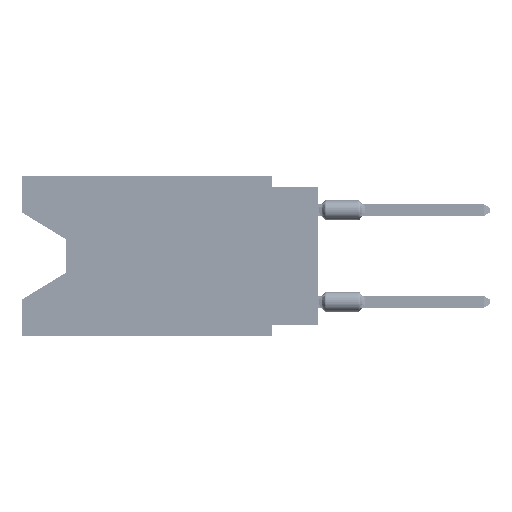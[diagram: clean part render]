
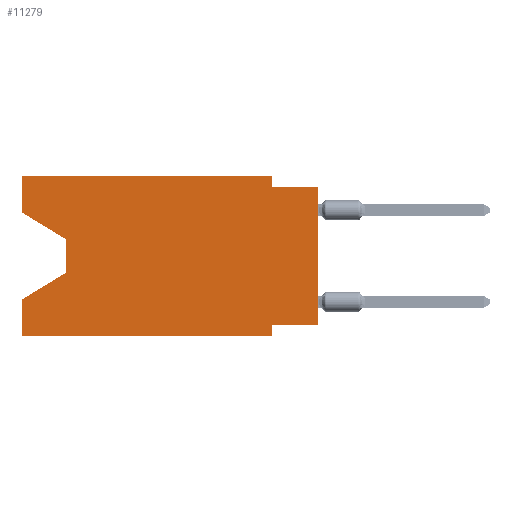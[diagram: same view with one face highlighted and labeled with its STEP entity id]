
A CAD part, left-side view. The second image highlights one B-rep face of the part: STEP entity #11279.
In plain terms, the highlighted planar face has unit normal (-1, 0, 0).
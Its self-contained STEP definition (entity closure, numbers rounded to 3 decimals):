
#950 = DIRECTION ( 'NONE',  ( 0., 0., 1. ) ) ;
#1279 = ORIENTED_EDGE ( 'NONE', *, *, #29455, .F. ) ;
#1303 = LINE ( 'NONE', #45888, #50963 ) ;
#3090 = CARTESIAN_POINT ( 'NONE',  ( 0., 16.383, -8.89 ) ) ;
#3572 = CARTESIAN_POINT ( 'NONE',  ( 0., 2.54, -8.89 ) ) ;
#4614 = VERTEX_POINT ( 'NONE', #33083 ) ;
#5511 = VECTOR ( 'NONE', #44005, 1000. ) ;
#6812 = CARTESIAN_POINT ( 'NONE',  ( 0., 0., -0.635 ) ) ;
#6932 = CARTESIAN_POINT ( 'NONE',  ( 0., 2.54, -8.89 ) ) ;
#8060 = EDGE_CURVE ( 'NONE', #33453, #52385, #30793, .T. ) ;
#8315 = LINE ( 'NONE', #13785, #61942 ) ;
#8865 = VECTOR ( 'NONE', #48893, 1000. ) ;
#9312 = VECTOR ( 'NONE', #46391, 1000. ) ;
#9789 = EDGE_CURVE ( 'NONE', #4614, #21553, #8315, .T. ) ;
#11019 = ORIENTED_EDGE ( 'NONE', *, *, #30261, .F. ) ;
#11279 = ADVANCED_FACE ( 'NONE', ( #70111 ), #65358, .F. ) ;
#13785 = CARTESIAN_POINT ( 'NONE',  ( 0., 16.383, -2.038 ) ) ;
#13865 = LINE ( 'NONE', #70539, #41864 ) ;
#14086 = EDGE_CURVE ( 'NONE', #66537, #68276, #41942, .T. ) ;
#14287 = DIRECTION ( 'NONE',  ( 0., 0., 1. ) ) ;
#15122 = CARTESIAN_POINT ( 'NONE',  ( 0., 16.383, 0. ) ) ;
#15493 = LINE ( 'NONE', #59031, #36379 ) ;
#15841 = LINE ( 'NONE', #71785, #44461 ) ;
#16662 = AXIS2_PLACEMENT_3D ( 'NONE', #71562, #37548, #26945 ) ;
#17237 = LINE ( 'NONE', #39890, #37788 ) ;
#18058 = LINE ( 'NONE', #53416, #25051 ) ;
#18403 = ORIENTED_EDGE ( 'NONE', *, *, #62581, .F. ) ;
#18841 = LINE ( 'NONE', #63453, #46507 ) ;
#19625 = VERTEX_POINT ( 'NONE', #66062 ) ;
#21553 = VERTEX_POINT ( 'NONE', #54909 ) ;
#21654 = ORIENTED_EDGE ( 'NONE', *, *, #52758, .F. ) ;
#21804 = CARTESIAN_POINT ( 'NONE',  ( 0., 13.97, -5.385 ) ) ;
#23381 = LINE ( 'NONE', #67645, #9312 ) ;
#24549 = VECTOR ( 'NONE', #53854, 1000. ) ;
#25051 = VECTOR ( 'NONE', #14287, 1000. ) ;
#25361 = DIRECTION ( 'NONE',  ( 0., 0., -1. ) ) ;
#26404 = VERTEX_POINT ( 'NONE', #3090 ) ;
#26851 = ORIENTED_EDGE ( 'NONE', *, *, #43022, .T. ) ;
#26939 = CARTESIAN_POINT ( 'NONE',  ( 0., 16.383, -6.852 ) ) ;
#26945 = DIRECTION ( 'NONE',  ( 0., 0., -1. ) ) ;
#28386 = ORIENTED_EDGE ( 'NONE', *, *, #14086, .F. ) ;
#28554 = VERTEX_POINT ( 'NONE', #26939 ) ;
#28732 = EDGE_CURVE ( 'NONE', #42422, #52385, #18841, .T. ) ;
#29455 = EDGE_CURVE ( 'NONE', #60139, #19625, #13865, .T. ) ;
#30261 = EDGE_CURVE ( 'NONE', #19625, #33453, #23381, .T. ) ;
#30793 = LINE ( 'NONE', #6812, #24549 ) ;
#33083 = CARTESIAN_POINT ( 'NONE',  ( 0., 16.383, -2.038 ) ) ;
#33453 = VERTEX_POINT ( 'NONE', #35591 ) ;
#34282 = VERTEX_POINT ( 'NONE', #21804 ) ;
#34705 = ORIENTED_EDGE ( 'NONE', *, *, #71980, .T. ) ;
#35591 = CARTESIAN_POINT ( 'NONE',  ( 0., 2.54, -0.635 ) ) ;
#36379 = VECTOR ( 'NONE', #25361, 1000. ) ;
#36411 = EDGE_CURVE ( 'NONE', #26404, #68276, #17237, .T. ) ;
#37548 = DIRECTION ( 'NONE',  ( 1., 0., 0. ) ) ;
#37788 = VECTOR ( 'NONE', #57103, 1000. ) ;
#38464 = CARTESIAN_POINT ( 'NONE',  ( 0., 2.54, -8.255 ) ) ;
#38511 = LINE ( 'NONE', #65253, #5511 ) ;
#39890 = CARTESIAN_POINT ( 'NONE',  ( 0., 16.383, -8.89 ) ) ;
#41864 = VECTOR ( 'NONE', #69451, 1000. ) ;
#41942 = LINE ( 'NONE', #3572, #8865 ) ;
#42422 = VERTEX_POINT ( 'NONE', #68024 ) ;
#43022 = EDGE_CURVE ( 'NONE', #34282, #28554, #38511, .T. ) ;
#44005 = DIRECTION ( 'NONE',  ( 0., 0.855, -0.519 ) ) ;
#44461 = VECTOR ( 'NONE', #55701, 1000. ) ;
#45888 = CARTESIAN_POINT ( 'NONE',  ( 0., 0., -8.255 ) ) ;
#46391 = DIRECTION ( 'NONE',  ( 0., 0., -1. ) ) ;
#46507 = VECTOR ( 'NONE', #950, 1000. ) ;
#46992 = ORIENTED_EDGE ( 'NONE', *, *, #36411, .T. ) ;
#47183 = EDGE_CURVE ( 'NONE', #4614, #60139, #15841, .T. ) ;
#47231 = ORIENTED_EDGE ( 'NONE', *, *, #8060, .F. ) ;
#48893 = DIRECTION ( 'NONE',  ( 0., 0., -1. ) ) ;
#50963 = VECTOR ( 'NONE', #68210, 1000. ) ;
#52385 = VERTEX_POINT ( 'NONE', #59495 ) ;
#52562 = DIRECTION ( 'NONE',  ( 0., -0.855, -0.519 ) ) ;
#52758 = EDGE_CURVE ( 'NONE', #42422, #66537, #1303, .T. ) ;
#53416 = CARTESIAN_POINT ( 'NONE',  ( 0., 16.383, 0. ) ) ;
#53854 = DIRECTION ( 'NONE',  ( 0., -1., 0. ) ) ;
#53979 = ORIENTED_EDGE ( 'NONE', *, *, #9789, .T. ) ;
#54909 = CARTESIAN_POINT ( 'NONE',  ( 0., 13.97, -3.505 ) ) ;
#55701 = DIRECTION ( 'NONE',  ( 0., 0., 1. ) ) ;
#57103 = DIRECTION ( 'NONE',  ( 0., -1., 0. ) ) ;
#57402 = ORIENTED_EDGE ( 'NONE', *, *, #47183, .F. ) ;
#59031 = CARTESIAN_POINT ( 'NONE',  ( 0., 13.97, -3.505 ) ) ;
#59495 = CARTESIAN_POINT ( 'NONE',  ( 0., 0., -0.635 ) ) ;
#60139 = VERTEX_POINT ( 'NONE', #15122 ) ;
#60434 = EDGE_LOOP ( 'NONE', ( #53979, #34705, #26851, #18403, #46992, #28386, #21654, #67705, #47231, #11019, #1279, #57402 ) ) ;
#61942 = VECTOR ( 'NONE', #52562, 1000. ) ;
#62581 = EDGE_CURVE ( 'NONE', #26404, #28554, #18058, .T. ) ;
#63453 = CARTESIAN_POINT ( 'NONE',  ( 0., 0., 0. ) ) ;
#65253 = CARTESIAN_POINT ( 'NONE',  ( 0., 13.97, -5.385 ) ) ;
#65358 = PLANE ( 'NONE',  #16662 ) ;
#66062 = CARTESIAN_POINT ( 'NONE',  ( 0., 2.54, 0. ) ) ;
#66537 = VERTEX_POINT ( 'NONE', #38464 ) ;
#67645 = CARTESIAN_POINT ( 'NONE',  ( 0., 2.54, 0. ) ) ;
#67705 = ORIENTED_EDGE ( 'NONE', *, *, #28732, .T. ) ;
#68024 = CARTESIAN_POINT ( 'NONE',  ( 0., 0., -8.255 ) ) ;
#68210 = DIRECTION ( 'NONE',  ( 0., 1., 0. ) ) ;
#68276 = VERTEX_POINT ( 'NONE', #6932 ) ;
#69451 = DIRECTION ( 'NONE',  ( 0., -1., 0. ) ) ;
#70111 = FACE_OUTER_BOUND ( 'NONE', #60434, .T. ) ;
#70539 = CARTESIAN_POINT ( 'NONE',  ( 0., 16.383, 0. ) ) ;
#71562 = CARTESIAN_POINT ( 'NONE',  ( 0., 16.383, 0. ) ) ;
#71785 = CARTESIAN_POINT ( 'NONE',  ( 0., 16.383, 0. ) ) ;
#71980 = EDGE_CURVE ( 'NONE', #21553, #34282, #15493, .T. ) ;
